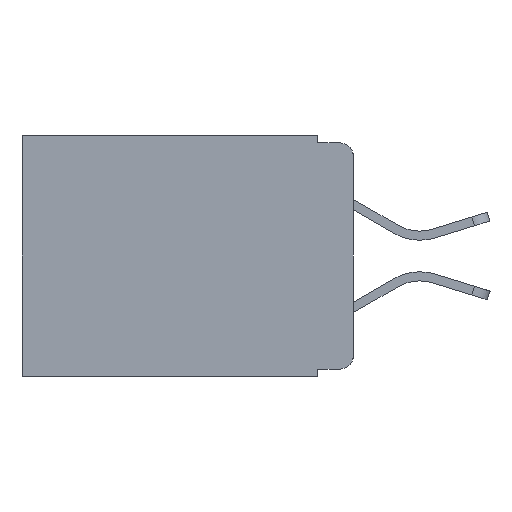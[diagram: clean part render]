
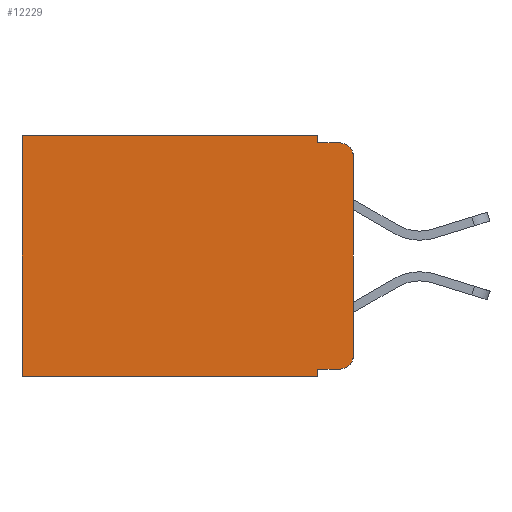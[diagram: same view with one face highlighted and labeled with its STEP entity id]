
A CAD part, left-side view. The second image highlights one B-rep face of the part: STEP entity #12229.
In plain terms, the highlighted planar face has unit normal (-1, 0, 0).
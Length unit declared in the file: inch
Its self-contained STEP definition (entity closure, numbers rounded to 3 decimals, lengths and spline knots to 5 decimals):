
#15 = CARTESIAN_POINT ( 'NONE',  ( 0.298, 0.051, -0.333 ) ) ;
#220 = ORIENTED_EDGE ( 'NONE', *, *, #755, .F. ) ;
#252 = ORIENTED_EDGE ( 'NONE', *, *, #7157, .T. ) ;
#334 = CARTESIAN_POINT ( 'NONE',  ( 0.298, 0.051, 0. ) ) ;
#362 = CIRCLE ( 'NONE', #11588, 0.02 ) ;
#425 = CARTESIAN_POINT ( 'NONE',  ( 0.298, 0.051, -0.343 ) ) ;
#605 = CARTESIAN_POINT ( 'NONE',  ( 0.298, 0., 0. ) ) ;
#755 = EDGE_CURVE ( 'NONE', #11598, #5788, #9842, .T. ) ;
#811 = DIRECTION ( 'NONE',  ( 0., -1., 0. ) ) ;
#1129 = CARTESIAN_POINT ( 'NONE',  ( 0.298, 0.051, 0. ) ) ;
#1259 = LINE ( 'NONE', #1739, #2695 ) ;
#1352 = VERTEX_POINT ( 'NONE', #1129 ) ;
#1739 = CARTESIAN_POINT ( 'NONE',  ( 0.298, 0.051, 0. ) ) ;
#1870 = EDGE_CURVE ( 'NONE', #4398, #2363, #14165, .T. ) ;
#1922 = CARTESIAN_POINT ( 'NONE',  ( 0.298, 0.051, -0.01 ) ) ;
#2159 = ORIENTED_EDGE ( 'NONE', *, *, #8272, .T. ) ;
#2228 = CARTESIAN_POINT ( 'NONE',  ( 0.298, 0.02, -0.313 ) ) ;
#2332 = LINE ( 'NONE', #2614, #14294 ) ;
#2363 = VERTEX_POINT ( 'NONE', #8259 ) ;
#2614 = CARTESIAN_POINT ( 'NONE',  ( 0.298, 0., -0.343 ) ) ;
#2695 = VECTOR ( 'NONE', #10793, 39.37008 ) ;
#2867 = VECTOR ( 'NONE', #10746, 39.37008 ) ;
#3122 = CARTESIAN_POINT ( 'NONE',  ( 0.298, 0.02, -0.333 ) ) ;
#3801 = DIRECTION ( 'NONE',  ( 0., 1., 0. ) ) ;
#3852 = AXIS2_PLACEMENT_3D ( 'NONE', #2228, #12648, #5767 ) ;
#3944 = VERTEX_POINT ( 'NONE', #3122 ) ;
#3970 = VECTOR ( 'NONE', #811, 39.37008 ) ;
#4398 = VERTEX_POINT ( 'NONE', #6487 ) ;
#4725 = CARTESIAN_POINT ( 'NONE',  ( 0.298, 0., -0.313 ) ) ;
#5190 = LINE ( 'NONE', #7960, #8466 ) ;
#5263 = VERTEX_POINT ( 'NONE', #425 ) ;
#5314 = PLANE ( 'NONE',  #5334 ) ;
#5334 = AXIS2_PLACEMENT_3D ( 'NONE', #11306, #6488, #10184 ) ;
#5539 = EDGE_CURVE ( 'NONE', #1352, #4398, #11228, .T. ) ;
#5767 = DIRECTION ( 'NONE',  ( 0., 0., -1. ) ) ;
#5788 = VERTEX_POINT ( 'NONE', #4725 ) ;
#6086 = EDGE_CURVE ( 'NONE', #11598, #9909, #362, .T. ) ;
#6142 = FACE_OUTER_BOUND ( 'NONE', #12479, .T. ) ;
#6349 = EDGE_CURVE ( 'NONE', #8307, #5263, #9757, .T. ) ;
#6429 = EDGE_CURVE ( 'NONE', #1352, #14607, #1259, .T. ) ;
#6487 = CARTESIAN_POINT ( 'NONE',  ( 0.298, 0.473, 0. ) ) ;
#6488 = DIRECTION ( 'NONE',  ( 1., 0., 0. ) ) ;
#6577 = CARTESIAN_POINT ( 'NONE',  ( 0.298, 0.02, -0.03 ) ) ;
#6642 = ORIENTED_EDGE ( 'NONE', *, *, #5539, .T. ) ;
#6773 = ORIENTED_EDGE ( 'NONE', *, *, #6086, .T. ) ;
#7053 = LINE ( 'NONE', #1922, #3970 ) ;
#7157 = EDGE_CURVE ( 'NONE', #8307, #3944, #5190, .T. ) ;
#7757 = DIRECTION ( 'NONE',  ( -1., 0., 0. ) ) ;
#7819 = VECTOR ( 'NONE', #12771, 39.37008 ) ;
#7960 = CARTESIAN_POINT ( 'NONE',  ( 0.298, 0.051, -0.333 ) ) ;
#8027 = ORIENTED_EDGE ( 'NONE', *, *, #11364, .F. ) ;
#8259 = CARTESIAN_POINT ( 'NONE',  ( 0.298, 0.473, -0.343 ) ) ;
#8272 = EDGE_CURVE ( 'NONE', #3944, #5788, #8770, .T. ) ;
#8307 = VERTEX_POINT ( 'NONE', #15 ) ;
#8466 = VECTOR ( 'NONE', #10222, 39.37008 ) ;
#8508 = VECTOR ( 'NONE', #12129, 39.37008 ) ;
#8770 = CIRCLE ( 'NONE', #3852, 0.02 ) ;
#8970 = DIRECTION ( 'NONE',  ( 0., 0., -1. ) ) ;
#9302 = VECTOR ( 'NONE', #12183, 39.37008 ) ;
#9567 = CARTESIAN_POINT ( 'NONE',  ( 0.298, 0.051, -0.01 ) ) ;
#9757 = LINE ( 'NONE', #334, #2867 ) ;
#9842 = LINE ( 'NONE', #13419, #9302 ) ;
#9909 = VERTEX_POINT ( 'NONE', #14408 ) ;
#10184 = DIRECTION ( 'NONE',  ( 0., 0., -1. ) ) ;
#10222 = DIRECTION ( 'NONE',  ( 0., -1., 0. ) ) ;
#10746 = DIRECTION ( 'NONE',  ( 0., 0., -1. ) ) ;
#10793 = DIRECTION ( 'NONE',  ( 0., 0., -1. ) ) ;
#11228 = LINE ( 'NONE', #605, #8508 ) ;
#11306 = CARTESIAN_POINT ( 'NONE',  ( 0.298, 0., 0. ) ) ;
#11364 = EDGE_CURVE ( 'NONE', #14607, #9909, #7053, .T. ) ;
#11588 = AXIS2_PLACEMENT_3D ( 'NONE', #6577, #7757, #8970 ) ;
#11598 = VERTEX_POINT ( 'NONE', #14122 ) ;
#11676 = EDGE_CURVE ( 'NONE', #5263, #2363, #2332, .T. ) ;
#11713 = CARTESIAN_POINT ( 'NONE',  ( 0.298, 0.473, 0. ) ) ;
#12129 = DIRECTION ( 'NONE',  ( 0., 1., 0. ) ) ;
#12183 = DIRECTION ( 'NONE',  ( 0., 0., -1. ) ) ;
#12229 = ADVANCED_FACE ( 'NONE', ( #6142 ), #5314, .F. ) ;
#12479 = EDGE_LOOP ( 'NONE', ( #220, #6773, #8027, #13329, #6642, #14800, #13751, #13508, #252, #2159 ) ) ;
#12648 = DIRECTION ( 'NONE',  ( -1., 0., 0. ) ) ;
#12771 = DIRECTION ( 'NONE',  ( 0., 0., -1. ) ) ;
#13329 = ORIENTED_EDGE ( 'NONE', *, *, #6429, .F. ) ;
#13419 = CARTESIAN_POINT ( 'NONE',  ( 0.298, 0., 0. ) ) ;
#13508 = ORIENTED_EDGE ( 'NONE', *, *, #6349, .F. ) ;
#13751 = ORIENTED_EDGE ( 'NONE', *, *, #11676, .F. ) ;
#14122 = CARTESIAN_POINT ( 'NONE',  ( 0.298, 0., -0.03 ) ) ;
#14165 = LINE ( 'NONE', #11713, #7819 ) ;
#14294 = VECTOR ( 'NONE', #3801, 39.37008 ) ;
#14408 = CARTESIAN_POINT ( 'NONE',  ( 0.298, 0.02, -0.01 ) ) ;
#14607 = VERTEX_POINT ( 'NONE', #9567 ) ;
#14800 = ORIENTED_EDGE ( 'NONE', *, *, #1870, .T. ) ;
